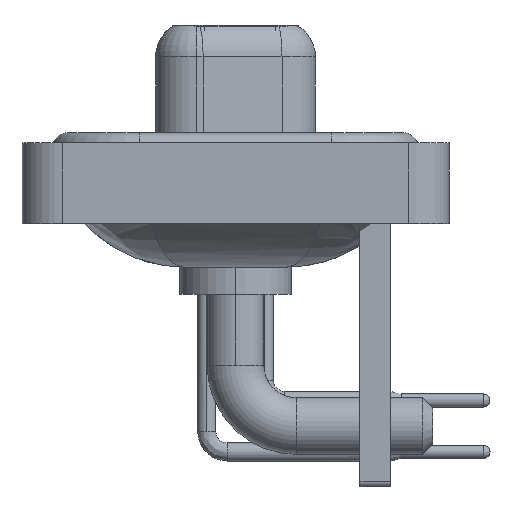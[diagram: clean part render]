
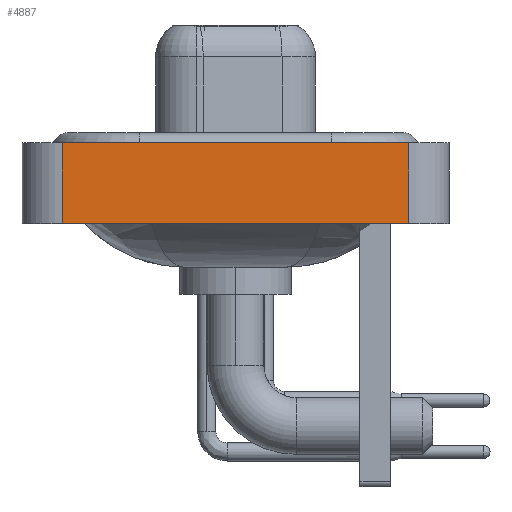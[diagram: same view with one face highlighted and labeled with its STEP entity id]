
A CAD part, left-side view. The second image highlights one B-rep face of the part: STEP entity #4887.
In plain terms, the highlighted planar face has unit normal (-1, 0, 0).
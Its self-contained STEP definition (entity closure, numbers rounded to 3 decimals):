
#317 = FACE_OUTER_BOUND ( 'NONE', #3663, .T. ) ;
#2909 = ORIENTED_EDGE ( 'NONE', *, *, #12209, .T. ) ;
#3364 = DIRECTION ( 'NONE',  ( 0., 0., 1. ) ) ;
#3663 = EDGE_LOOP ( 'NONE', ( #2909, #17148, #4384, #10801 ) ) ;
#4143 = DIRECTION ( 'NONE',  ( 0., -1., 0. ) ) ;
#4384 = ORIENTED_EDGE ( 'NONE', *, *, #24769, .F. ) ;
#4447 = VERTEX_POINT ( 'NONE', #17679 ) ;
#4887 = ADVANCED_FACE ( 'NONE', ( #317 ), #16230, .T. ) ;
#5186 = CARTESIAN_POINT ( 'NONE',  ( -7.35, -8.55, -3.6 ) ) ;
#5444 = CARTESIAN_POINT ( 'NONE',  ( -7.35, 8.55, -3.6 ) ) ;
#5943 = CARTESIAN_POINT ( 'NONE',  ( -7.35, -8.55, -3.6 ) ) ;
#6365 = VERTEX_POINT ( 'NONE', #23203 ) ;
#6476 = CARTESIAN_POINT ( 'NONE',  ( -7.35, -8.55, -3.6 ) ) ;
#7397 = CARTESIAN_POINT ( 'NONE',  ( -7.35, -8.55, -3.6 ) ) ;
#10317 = DIRECTION ( 'NONE',  ( -1., 0., 0. ) ) ;
#10801 = ORIENTED_EDGE ( 'NONE', *, *, #18431, .T. ) ;
#10970 = VERTEX_POINT ( 'NONE', #5186 ) ;
#12093 = LINE ( 'NONE', #5943, #19222 ) ;
#12209 = EDGE_CURVE ( 'NONE', #10970, #24725, #25009, .T. ) ;
#13048 = CARTESIAN_POINT ( 'NONE',  ( -7.35, -8.55, 0.4 ) ) ;
#13307 = DIRECTION ( 'NONE',  ( 0., -1., 0. ) ) ;
#14090 = EDGE_CURVE ( 'NONE', #6365, #24725, #14836, .T. ) ;
#14836 = LINE ( 'NONE', #13048, #23171 ) ;
#15213 = DIRECTION ( 'NONE',  ( 0., 0., 1. ) ) ;
#15977 = DIRECTION ( 'NONE',  ( 0., 0., 1. ) ) ;
#16152 = CARTESIAN_POINT ( 'NONE',  ( -7.35, -8.55, 0.4 ) ) ;
#16230 = PLANE ( 'NONE',  #17170 ) ;
#17112 = VECTOR ( 'NONE', #3364, 1000. ) ;
#17148 = ORIENTED_EDGE ( 'NONE', *, *, #14090, .F. ) ;
#17170 = AXIS2_PLACEMENT_3D ( 'NONE', #6476, #10317, #15977 ) ;
#17679 = CARTESIAN_POINT ( 'NONE',  ( -7.35, 8.55, -3.6 ) ) ;
#18264 = VECTOR ( 'NONE', #15213, 1000. ) ;
#18431 = EDGE_CURVE ( 'NONE', #4447, #10970, #12093, .T. ) ;
#19222 = VECTOR ( 'NONE', #4143, 1000. ) ;
#19464 = LINE ( 'NONE', #5444, #17112 ) ;
#23171 = VECTOR ( 'NONE', #13307, 1000. ) ;
#23203 = CARTESIAN_POINT ( 'NONE',  ( -7.35, 8.55, 0.4 ) ) ;
#24725 = VERTEX_POINT ( 'NONE', #16152 ) ;
#24769 = EDGE_CURVE ( 'NONE', #4447, #6365, #19464, .T. ) ;
#25009 = LINE ( 'NONE', #7397, #18264 ) ;
